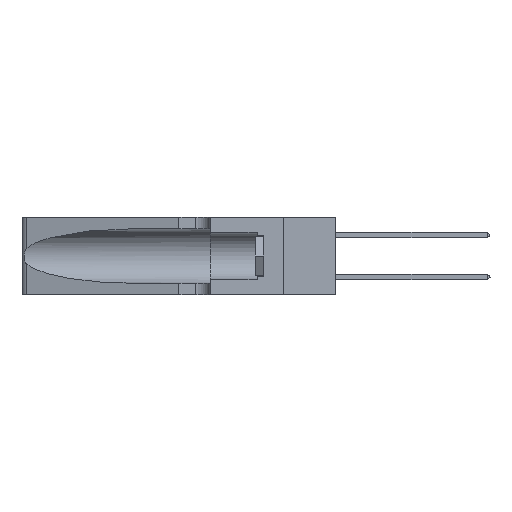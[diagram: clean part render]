
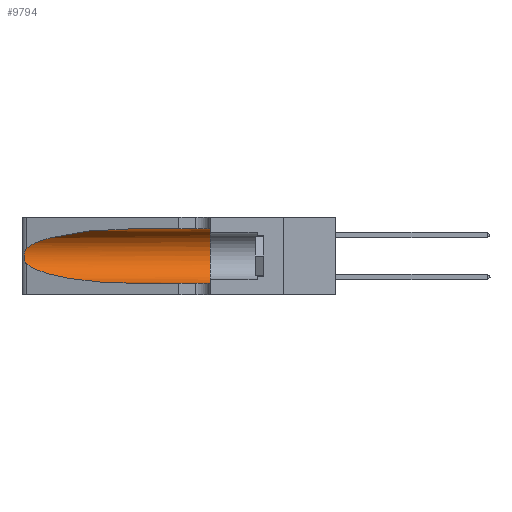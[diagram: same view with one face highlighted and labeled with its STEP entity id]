
A CAD part, left-side view. The second image highlights one B-rep face of the part: STEP entity #9794.
In plain terms, the highlighted cylindrical face has radius 3.308 mm (diameter 6.617 mm), a partial arc.
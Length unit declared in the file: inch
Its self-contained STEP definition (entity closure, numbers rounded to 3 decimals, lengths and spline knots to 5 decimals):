
#2041 = CIRCLE ( 'NONE', #28314, 0.13025 ) ;
#2215 = CARTESIAN_POINT ( 'NONE',  ( 0.18966, 0.96281, 0.31525 ) ) ;
#3316 = VECTOR ( 'NONE', #8731, 39.37008 ) ;
#3418 = CARTESIAN_POINT ( 'NONE',  ( 0.25854, 1.2359, 0.20912 ) ) ;
#5205 = CARTESIAN_POINT ( 'NONE',  ( 0.1305, 0.72297, 0.05475 ) ) ;
#5460 = CARTESIAN_POINT ( 'NONE',  ( 0.26075, 1.23896, 0.19203 ) ) ;
#5669 = CARTESIAN_POINT ( 'NONE',  ( 0.25787, 1.23484, 0.2124 ) ) ;
#5928 = CARTESIAN_POINT ( 'NONE',  ( 0.18966, 0.96281, 0.05475 ) ) ;
#7316 =( BOUNDED_CURVE ( )  B_SPLINE_CURVE ( 3, ( #13819, #2215, #9428, #18426 ),
 .UNSPECIFIED., .F., .F. ) 
 B_SPLINE_CURVE_WITH_KNOTS ( ( 4, 4 ),
 ( 1.5708, 2.84003 ),
 .UNSPECIFIED. ) 
 CURVE ( )  GEOMETRIC_REPRESENTATION_ITEM ( )  RATIONAL_B_SPLINE_CURVE ( ( 1., 0.87, 0.87, 1. ) ) 
 REPRESENTATION_ITEM ( '' )  );
#7689 = CARTESIAN_POINT ( 'NONE',  ( 0.25487, 1.22718, 0.14631 ) ) ;
#7798 = EDGE_CURVE ( 'NONE', #9970, #22848, #16399, .T. ) ;
#8066 = ORIENTED_EDGE ( 'NONE', *, *, #9251, .T. ) ;
#8106 = CARTESIAN_POINT ( 'NONE',  ( 0.25555, 1.22994, 0.2215 ) ) ;
#8272 = B_SPLINE_CURVE_WITH_KNOTS ( 'NONE', 3,
 ( #23836, #8106, #26272, #5669, #3418, #26585, #5460, #12783, #26472, #21521, #23934, #17091, #28895, #7689 ),
 .UNSPECIFIED., .F., .F.,
 ( 4, 2, 2, 2, 2, 2, 4 ),
 ( 0., 0.00027, 0.00053, 0.00107, 0.0016, 0.00187, 0.00214 ),
 .UNSPECIFIED. ) ;
#8339 = ORIENTED_EDGE ( 'NONE', *, *, #19617, .T. ) ;
#8731 = DIRECTION ( 'NONE',  ( 0., -1., 0. ) ) ;
#9196 = CARTESIAN_POINT ( 'NONE',  ( 0.25487, 1.22718, 0.14631 ) ) ;
#9251 = EDGE_CURVE ( 'NONE', #9970, #15349, #7316, .T. ) ;
#9428 = CARTESIAN_POINT ( 'NONE',  ( 0.2373, 1.15595, 0.28018 ) ) ;
#9685 = DIRECTION ( 'NONE',  ( 0., 0., -1. ) ) ;
#9780 = DIRECTION ( 'NONE',  ( 0., -1., 0. ) ) ;
#9794 = ADVANCED_FACE ( 'NONE', ( #21275 ), #10878, .F. ) ;
#9970 = VERTEX_POINT ( 'NONE', #19570 ) ;
#10562 = VERTEX_POINT ( 'NONE', #20518 ) ;
#10591 = CARTESIAN_POINT ( 'NONE',  ( 0.25487, 1.22718, 0.22369 ) ) ;
#10796 = DIRECTION ( 'NONE',  ( 0., 1., 0. ) ) ;
#10878 = CYLINDRICAL_SURFACE ( 'NONE', #21887, 0.13025 ) ;
#10989 = CARTESIAN_POINT ( 'NONE',  ( 0.1305, 1.61858, 0.31525 ) ) ;
#11055 = CARTESIAN_POINT ( 'NONE',  ( 0.1305, 0.35, 0.31525 ) ) ;
#11058 = VECTOR ( 'NONE', #19687, 39.37008 ) ;
#11927 = ORIENTED_EDGE ( 'NONE', *, *, #22681, .T. ) ;
#11967 = ORIENTED_EDGE ( 'NONE', *, *, #26716, .F. ) ;
#11979 = VERTEX_POINT ( 'NONE', #5205 ) ;
#12783 = CARTESIAN_POINT ( 'NONE',  ( 0.26075, 1.23896, 0.178 ) ) ;
#13819 = CARTESIAN_POINT ( 'NONE',  ( 0.1305, 0.72297, 0.31525 ) ) ;
#15027 = DIRECTION ( 'NONE',  ( 0., 0., 1. ) ) ;
#15349 = VERTEX_POINT ( 'NONE', #10591 ) ;
#16399 = LINE ( 'NONE', #10989, #3316 ) ;
#17091 = CARTESIAN_POINT ( 'NONE',  ( 0.25639, 1.23186, 0.15144 ) ) ;
#17311 = EDGE_LOOP ( 'NONE', ( #8066, #25349, #8339, #11927, #11967, #28959 ) ) ;
#18426 = CARTESIAN_POINT ( 'NONE',  ( 0.25487, 1.22718, 0.22369 ) ) ;
#18623 =( BOUNDED_CURVE ( )  B_SPLINE_CURVE ( 3, ( #24296, #19752, #5928, #27319 ),
 .UNSPECIFIED., .F., .F. ) 
 B_SPLINE_CURVE_WITH_KNOTS ( ( 4, 4 ),
 ( 3.44316, 4.71239 ),
 .UNSPECIFIED. ) 
 CURVE ( )  GEOMETRIC_REPRESENTATION_ITEM ( )  RATIONAL_B_SPLINE_CURVE ( ( 1., 0.87, 0.87, 1. ) ) 
 REPRESENTATION_ITEM ( '' )  );
#19570 = CARTESIAN_POINT ( 'NONE',  ( 0.1305, 0.72297, 0.31525 ) ) ;
#19617 = EDGE_CURVE ( 'NONE', #25503, #11979, #18623, .T. ) ;
#19687 = DIRECTION ( 'NONE',  ( 0., -1., 0. ) ) ;
#19752 = CARTESIAN_POINT ( 'NONE',  ( 0.2373, 1.15595, 0.08982 ) ) ;
#20405 = LINE ( 'NONE', #28864, #11058 ) ;
#20518 = CARTESIAN_POINT ( 'NONE',  ( 0.1305, 0.35, 0.05475 ) ) ;
#21275 = FACE_OUTER_BOUND ( 'NONE', #17311, .T. ) ;
#21521 = CARTESIAN_POINT ( 'NONE',  ( 0.25856, 1.23593, 0.16098 ) ) ;
#21887 = AXIS2_PLACEMENT_3D ( 'NONE', #23614, #9780, #9685 ) ;
#22681 = EDGE_CURVE ( 'NONE', #11979, #10562, #20405, .T. ) ;
#22848 = VERTEX_POINT ( 'NONE', #11055 ) ;
#23614 = CARTESIAN_POINT ( 'NONE',  ( 0.1305, 1.61858, 0.185 ) ) ;
#23836 = CARTESIAN_POINT ( 'NONE',  ( 0.25487, 1.22718, 0.22369 ) ) ;
#23934 = CARTESIAN_POINT ( 'NONE',  ( 0.25789, 1.23486, 0.15765 ) ) ;
#24296 = CARTESIAN_POINT ( 'NONE',  ( 0.25487, 1.22718, 0.14631 ) ) ;
#25349 = ORIENTED_EDGE ( 'NONE', *, *, #28890, .T. ) ;
#25503 = VERTEX_POINT ( 'NONE', #9196 ) ;
#26272 = CARTESIAN_POINT ( 'NONE',  ( 0.25639, 1.23184, 0.21858 ) ) ;
#26472 = CARTESIAN_POINT ( 'NONE',  ( 0.26017, 1.23833, 0.17102 ) ) ;
#26585 = CARTESIAN_POINT ( 'NONE',  ( 0.26018, 1.23835, 0.19895 ) ) ;
#26716 = EDGE_CURVE ( 'NONE', #22848, #10562, #2041, .T. ) ;
#27319 = CARTESIAN_POINT ( 'NONE',  ( 0.1305, 0.72297, 0.05475 ) ) ;
#28314 = AXIS2_PLACEMENT_3D ( 'NONE', #28810, #10796, #15027 ) ;
#28810 = CARTESIAN_POINT ( 'NONE',  ( 0.1305, 0.35, 0.185 ) ) ;
#28864 = CARTESIAN_POINT ( 'NONE',  ( 0.1305, 1.61858, 0.05475 ) ) ;
#28890 = EDGE_CURVE ( 'NONE', #15349, #25503, #8272, .T. ) ;
#28895 = CARTESIAN_POINT ( 'NONE',  ( 0.25555, 1.22993, 0.14849 ) ) ;
#28959 = ORIENTED_EDGE ( 'NONE', *, *, #7798, .F. ) ;
